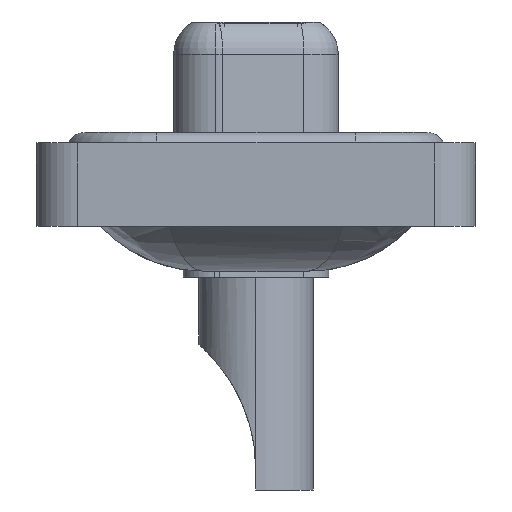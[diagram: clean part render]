
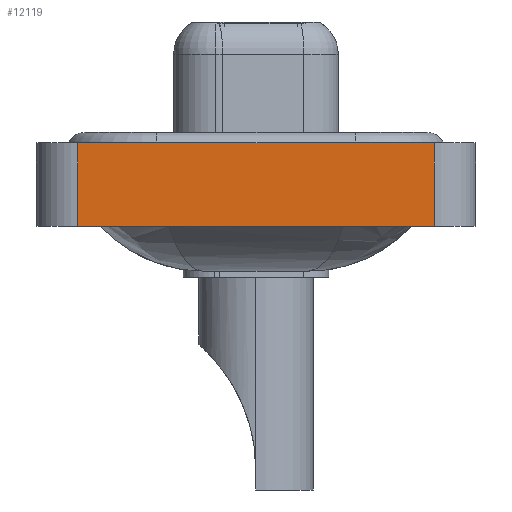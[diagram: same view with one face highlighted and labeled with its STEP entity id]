
A CAD part, left-side view. The second image highlights one B-rep face of the part: STEP entity #12119.
In plain terms, the highlighted planar face has unit normal (-1, 0, 0).
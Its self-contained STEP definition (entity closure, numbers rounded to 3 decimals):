
#60 = EDGE_CURVE ( 'NONE', #13173, #11262, #4019, .T. ) ;
#197 = CARTESIAN_POINT ( 'NONE',  ( -7.35, -8.55, -3.6 ) ) ;
#261 = VECTOR ( 'NONE', #12057, 1000. ) ;
#1282 = EDGE_LOOP ( 'NONE', ( #15952, #13942, #9179, #6767 ) ) ;
#1382 = VERTEX_POINT ( 'NONE', #12328 ) ;
#3223 = FACE_OUTER_BOUND ( 'NONE', #1282, .T. ) ;
#3820 = CARTESIAN_POINT ( 'NONE',  ( -7.35, -8.55, -3.6 ) ) ;
#4019 = LINE ( 'NONE', #6321, #11765 ) ;
#4478 = VECTOR ( 'NONE', #13025, 1000. ) ;
#4892 = CARTESIAN_POINT ( 'NONE',  ( -7.35, 8.55, 0.4 ) ) ;
#5699 = PLANE ( 'NONE',  #6125 ) ;
#5799 = VERTEX_POINT ( 'NONE', #14317 ) ;
#6111 = VECTOR ( 'NONE', #14545, 1000. ) ;
#6125 = AXIS2_PLACEMENT_3D ( 'NONE', #8510, #9764, #13707 ) ;
#6321 = CARTESIAN_POINT ( 'NONE',  ( -7.35, -8.55, 0.4 ) ) ;
#6407 = EDGE_CURVE ( 'NONE', #1382, #13173, #6854, .T. ) ;
#6470 = LINE ( 'NONE', #197, #6111 ) ;
#6767 = ORIENTED_EDGE ( 'NONE', *, *, #16064, .T. ) ;
#6854 = LINE ( 'NONE', #16111, #261 ) ;
#8510 = CARTESIAN_POINT ( 'NONE',  ( -7.35, -8.55, -3.6 ) ) ;
#9179 = ORIENTED_EDGE ( 'NONE', *, *, #6407, .F. ) ;
#9764 = DIRECTION ( 'NONE',  ( -1., 0., 0. ) ) ;
#10701 = LINE ( 'NONE', #3820, #4478 ) ;
#11262 = VERTEX_POINT ( 'NONE', #12225 ) ;
#11765 = VECTOR ( 'NONE', #14319, 1000. ) ;
#11849 = EDGE_CURVE ( 'NONE', #5799, #11262, #6470, .T. ) ;
#12057 = DIRECTION ( 'NONE',  ( 0., 0., 1. ) ) ;
#12119 = ADVANCED_FACE ( 'NONE', ( #3223 ), #5699, .T. ) ;
#12225 = CARTESIAN_POINT ( 'NONE',  ( -7.35, -8.55, 0.4 ) ) ;
#12328 = CARTESIAN_POINT ( 'NONE',  ( -7.35, 8.55, -3.6 ) ) ;
#13025 = DIRECTION ( 'NONE',  ( 0., -1., 0. ) ) ;
#13173 = VERTEX_POINT ( 'NONE', #4892 ) ;
#13707 = DIRECTION ( 'NONE',  ( 0., 0., 1. ) ) ;
#13942 = ORIENTED_EDGE ( 'NONE', *, *, #60, .F. ) ;
#14317 = CARTESIAN_POINT ( 'NONE',  ( -7.35, -8.55, -3.6 ) ) ;
#14319 = DIRECTION ( 'NONE',  ( 0., -1., 0. ) ) ;
#14545 = DIRECTION ( 'NONE',  ( 0., 0., 1. ) ) ;
#15952 = ORIENTED_EDGE ( 'NONE', *, *, #11849, .T. ) ;
#16064 = EDGE_CURVE ( 'NONE', #1382, #5799, #10701, .T. ) ;
#16111 = CARTESIAN_POINT ( 'NONE',  ( -7.35, 8.55, -3.6 ) ) ;
